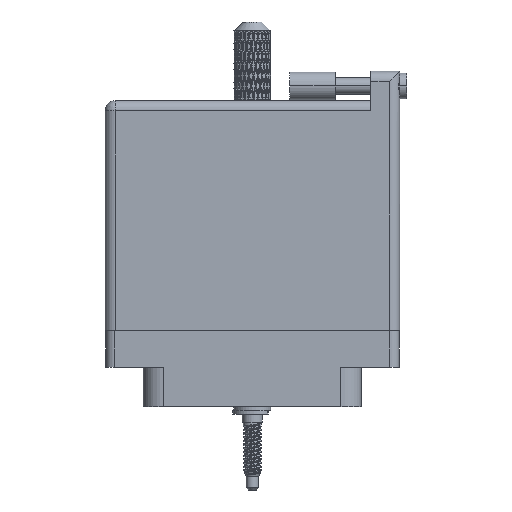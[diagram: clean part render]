
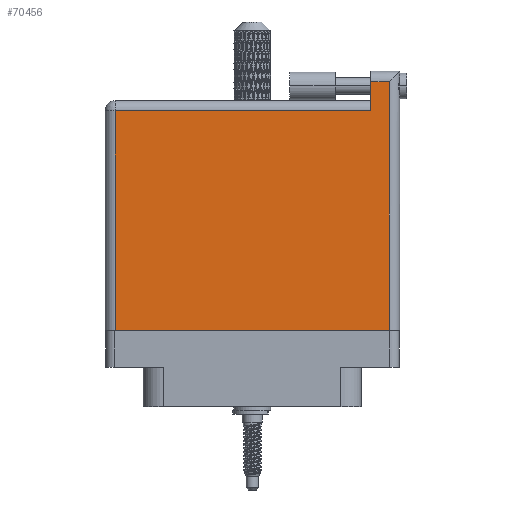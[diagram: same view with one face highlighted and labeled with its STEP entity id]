
A CAD part, front view. The second image highlights one B-rep face of the part: STEP entity #70456.
In plain terms, the highlighted face is planar.
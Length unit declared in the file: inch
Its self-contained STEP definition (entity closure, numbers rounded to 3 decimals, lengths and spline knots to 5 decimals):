
#224 = VERTEX_POINT ( 'NONE', #69396 ) ;
#1174 = FACE_OUTER_BOUND ( 'NONE', #98196, .T. ) ;
#6262 = CARTESIAN_POINT ( 'NONE',  ( -0.934, -0.1, 0.4495 ) ) ;
#6494 = DIRECTION ( 'NONE',  ( -1., 0., 0. ) ) ;
#7044 = CARTESIAN_POINT ( 'NONE',  ( 0.807, 1.396, 0.4495 ) ) ;
#9237 = CARTESIAN_POINT ( 'NONE',  ( 0.934, -0.1, 0.4495 ) ) ;
#15722 = VECTOR ( 'NONE', #92854, 39.37008 ) ;
#19359 = EDGE_CURVE ( 'NONE', #27869, #19648, #71466, .T. ) ;
#19648 = VERTEX_POINT ( 'NONE', #9237 ) ;
#22366 = DIRECTION ( 'NONE',  ( 0., -1., 0. ) ) ;
#22929 = PLANE ( 'NONE',  #23681 ) ;
#23409 = ORIENTED_EDGE ( 'NONE', *, *, #19359, .T. ) ;
#23681 = AXIS2_PLACEMENT_3D ( 'NONE', #79832, #31111, #6494 ) ;
#26346 = EDGE_CURVE ( 'NONE', #44998, #27869, #89414, .T. ) ;
#26527 = LINE ( 'NONE', #55931, #104220 ) ;
#27784 = CARTESIAN_POINT ( 'NONE',  ( -1.004, 1.596, 0.4495 ) ) ;
#27869 = VERTEX_POINT ( 'NONE', #105494 ) ;
#27994 = LINE ( 'NONE', #74852, #55884 ) ;
#28204 = VECTOR ( 'NONE', #32274, 39.37008 ) ;
#29612 = EDGE_CURVE ( 'NONE', #224, #76329, #27994, .T. ) ;
#31111 = DIRECTION ( 'NONE',  ( 0., 0., -1. ) ) ;
#32274 = DIRECTION ( 'NONE',  ( 1., 0., 0. ) ) ;
#35043 = ORIENTED_EDGE ( 'NONE', *, *, #93318, .T. ) ;
#41765 = ORIENTED_EDGE ( 'NONE', *, *, #29612, .T. ) ;
#43311 = ORIENTED_EDGE ( 'NONE', *, *, #52571, .T. ) ;
#44320 = VERTEX_POINT ( 'NONE', #70301 ) ;
#44998 = VERTEX_POINT ( 'NONE', #77120 ) ;
#49623 = CARTESIAN_POINT ( 'NONE',  ( -1.004, -0.1, 0.4495 ) ) ;
#52021 = DIRECTION ( 'NONE',  ( 0., -1., 0. ) ) ;
#52571 = EDGE_CURVE ( 'NONE', #19648, #44320, #84128, .T. ) ;
#53841 = LINE ( 'NONE', #27784, #15722 ) ;
#55884 = VECTOR ( 'NONE', #52021, 39.37008 ) ;
#55931 = CARTESIAN_POINT ( 'NONE',  ( -1.004, 1.396, 0.4495 ) ) ;
#57947 = CARTESIAN_POINT ( 'NONE',  ( 0.934, 1.666, 0.4495 ) ) ;
#58625 = DIRECTION ( 'NONE',  ( 0., 1., 0. ) ) ;
#64496 = DIRECTION ( 'NONE',  ( -1., 0., 0. ) ) ;
#69396 = CARTESIAN_POINT ( 'NONE',  ( 0.807, 1.596, 0.4495 ) ) ;
#70301 = CARTESIAN_POINT ( 'NONE',  ( 0.934, 1.596, 0.4495 ) ) ;
#70456 = ADVANCED_FACE ( 'NONE', ( #1174 ), #22929, .F. ) ;
#71466 = LINE ( 'NONE', #49623, #28204 ) ;
#74852 = CARTESIAN_POINT ( 'NONE',  ( 0.807, 1.666, 0.4495 ) ) ;
#76329 = VERTEX_POINT ( 'NONE', #7044 ) ;
#77120 = CARTESIAN_POINT ( 'NONE',  ( -0.934, 1.396, 0.4495 ) ) ;
#79832 = CARTESIAN_POINT ( 'NONE',  ( -1.004, 1.466, 0.4495 ) ) ;
#84128 = LINE ( 'NONE', #57947, #103216 ) ;
#85658 = VECTOR ( 'NONE', #22366, 39.37008 ) ;
#88491 = EDGE_CURVE ( 'NONE', #76329, #44998, #26527, .T. ) ;
#88820 = ORIENTED_EDGE ( 'NONE', *, *, #88491, .T. ) ;
#89414 = LINE ( 'NONE', #6262, #85658 ) ;
#92710 = ORIENTED_EDGE ( 'NONE', *, *, #26346, .T. ) ;
#92854 = DIRECTION ( 'NONE',  ( -1., 0., 0. ) ) ;
#93318 = EDGE_CURVE ( 'NONE', #44320, #224, #53841, .T. ) ;
#98196 = EDGE_LOOP ( 'NONE', ( #23409, #43311, #35043, #41765, #88820, #92710 ) ) ;
#103216 = VECTOR ( 'NONE', #58625, 39.37008 ) ;
#104220 = VECTOR ( 'NONE', #64496, 39.37008 ) ;
#105494 = CARTESIAN_POINT ( 'NONE',  ( -0.934, -0.1, 0.4495 ) ) ;
